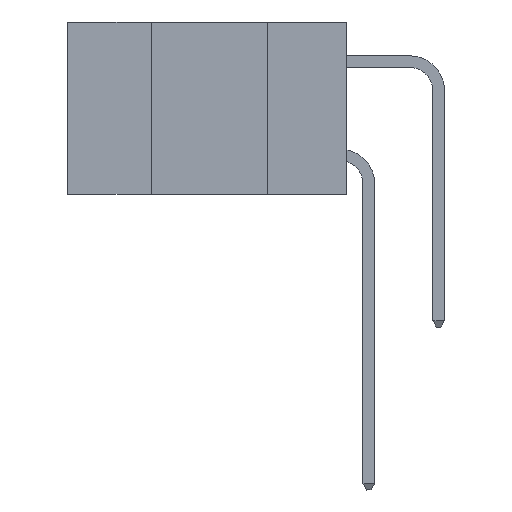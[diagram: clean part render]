
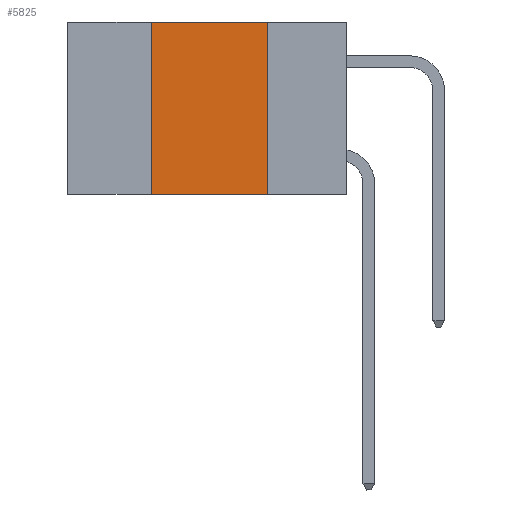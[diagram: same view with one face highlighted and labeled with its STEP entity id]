
A CAD part, left-side view. The second image highlights one B-rep face of the part: STEP entity #5825.
In plain terms, the highlighted planar face has unit normal (-1, 0, 0).
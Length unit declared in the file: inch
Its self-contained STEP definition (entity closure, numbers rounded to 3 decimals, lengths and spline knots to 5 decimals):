
#381 = DIRECTION ( 'NONE',  ( 0., 0., 1. ) ) ;
#448 = CARTESIAN_POINT ( 'NONE',  ( 0., 0.6, 0. ) ) ;
#485 = VERTEX_POINT ( 'NONE', #2586 ) ;
#742 = DIRECTION ( 'NONE',  ( 0., -1., 0. ) ) ;
#772 = LINE ( 'NONE', #9139, #9609 ) ;
#1243 = PLANE ( 'NONE',  #5888 ) ;
#1266 = VECTOR ( 'NONE', #9866, 39.37008 ) ;
#1340 = ORIENTED_EDGE ( 'NONE', *, *, #10277, .F. ) ;
#1637 = EDGE_CURVE ( 'NONE', #8900, #6801, #5155, .T. ) ;
#2586 = CARTESIAN_POINT ( 'NONE',  ( 0., 0.42, 0. ) ) ;
#4046 = CARTESIAN_POINT ( 'NONE',  ( 0., 0.42, -0.37 ) ) ;
#4627 = FACE_OUTER_BOUND ( 'NONE', #11175, .T. ) ;
#5037 = VERTEX_POINT ( 'NONE', #7901 ) ;
#5155 = LINE ( 'NONE', #6276, #6033 ) ;
#5214 = ORIENTED_EDGE ( 'NONE', *, *, #10926, .F. ) ;
#5571 = VECTOR ( 'NONE', #381, 39.37008 ) ;
#5825 = ADVANCED_FACE ( 'NONE', ( #4627 ), #1243, .F. ) ;
#5888 = AXIS2_PLACEMENT_3D ( 'NONE', #7838, #11463, #7809 ) ;
#6033 = VECTOR ( 'NONE', #742, 39.37008 ) ;
#6276 = CARTESIAN_POINT ( 'NONE',  ( 0., 0.6, -0.37 ) ) ;
#6563 = ORIENTED_EDGE ( 'NONE', *, *, #1637, .T. ) ;
#6801 = VERTEX_POINT ( 'NONE', #10778 ) ;
#7809 = DIRECTION ( 'NONE',  ( 0., 0., -1. ) ) ;
#7838 = CARTESIAN_POINT ( 'NONE',  ( 0., 0.6, 0. ) ) ;
#7901 = CARTESIAN_POINT ( 'NONE',  ( 0., 0.17, 0. ) ) ;
#8900 = VERTEX_POINT ( 'NONE', #4046 ) ;
#9136 = EDGE_CURVE ( 'NONE', #5037, #6801, #772, .T. ) ;
#9139 = CARTESIAN_POINT ( 'NONE',  ( 0., 0.17, 0. ) ) ;
#9609 = VECTOR ( 'NONE', #11002, 39.37008 ) ;
#9804 = LINE ( 'NONE', #448, #1266 ) ;
#9866 = DIRECTION ( 'NONE',  ( 0., -1., 0. ) ) ;
#10277 = EDGE_CURVE ( 'NONE', #485, #5037, #9804, .T. ) ;
#10778 = CARTESIAN_POINT ( 'NONE',  ( 0., 0.17, -0.37 ) ) ;
#10825 = ORIENTED_EDGE ( 'NONE', *, *, #9136, .F. ) ;
#10911 = LINE ( 'NONE', #11542, #5571 ) ;
#10926 = EDGE_CURVE ( 'NONE', #8900, #485, #10911, .T. ) ;
#11002 = DIRECTION ( 'NONE',  ( 0., 0., -1. ) ) ;
#11175 = EDGE_LOOP ( 'NONE', ( #10825, #1340, #5214, #6563 ) ) ;
#11463 = DIRECTION ( 'NONE',  ( 1., 0., 0. ) ) ;
#11542 = CARTESIAN_POINT ( 'NONE',  ( 0., 0.42, 0. ) ) ;
